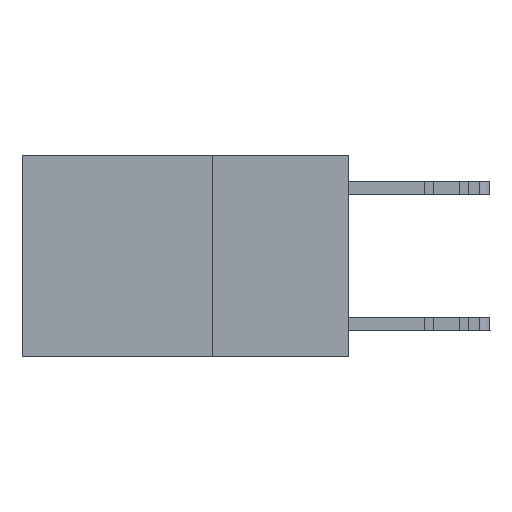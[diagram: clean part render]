
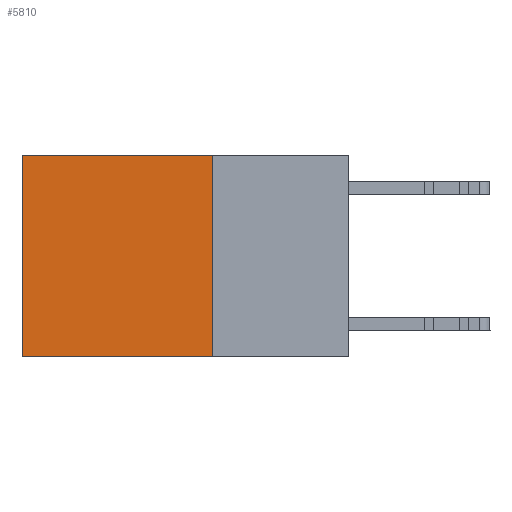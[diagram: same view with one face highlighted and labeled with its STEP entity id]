
A CAD part, left-side view. The second image highlights one B-rep face of the part: STEP entity #5810.
In plain terms, the highlighted planar face has unit normal (-1, 0, 0).
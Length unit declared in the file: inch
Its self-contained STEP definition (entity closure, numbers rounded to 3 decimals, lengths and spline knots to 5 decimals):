
#1325 = ORIENTED_EDGE ( 'NONE', *, *, #4437, .F. ) ;
#2714 = VERTEX_POINT ( 'NONE', #28033 ) ;
#4437 = EDGE_CURVE ( 'NONE', #5940, #8007, #23654, .T. ) ;
#5562 = CARTESIAN_POINT ( 'NONE',  ( 0.2625, 0.6, -0.37 ) ) ;
#5810 = ADVANCED_FACE ( 'NONE', ( #6890 ), #9930, .F. ) ;
#5861 = DIRECTION ( 'NONE',  ( 0., 0., -1. ) ) ;
#5940 = VERTEX_POINT ( 'NONE', #23942 ) ;
#6042 = DIRECTION ( 'NONE',  ( 1., 0., 0. ) ) ;
#6890 = FACE_OUTER_BOUND ( 'NONE', #17644, .T. ) ;
#8007 = VERTEX_POINT ( 'NONE', #5562 ) ;
#8303 = CARTESIAN_POINT ( 'NONE',  ( 0.2625, 0.25, 0. ) ) ;
#9930 = PLANE ( 'NONE',  #19287 ) ;
#10424 = LINE ( 'NONE', #21560, #10530 ) ;
#10530 = VECTOR ( 'NONE', #17144, 39.37008 ) ;
#12649 = EDGE_CURVE ( 'NONE', #2714, #5940, #20959, .T. ) ;
#12676 = VERTEX_POINT ( 'NONE', #23546 ) ;
#14909 = EDGE_CURVE ( 'NONE', #2714, #12676, #25557, .T. ) ;
#16536 = CARTESIAN_POINT ( 'NONE',  ( 0.2625, 0.25, -0.37 ) ) ;
#16691 = DIRECTION ( 'NONE',  ( 0., 1., 0. ) ) ;
#17123 = ORIENTED_EDGE ( 'NONE', *, *, #14909, .T. ) ;
#17144 = DIRECTION ( 'NONE',  ( 0., 0., -1. ) ) ;
#17644 = EDGE_LOOP ( 'NONE', ( #20929, #1325, #22571, #17123 ) ) ;
#18832 = DIRECTION ( 'NONE',  ( 0., 1., 0. ) ) ;
#18970 = CARTESIAN_POINT ( 'NONE',  ( 0.2625, 0.25, 0. ) ) ;
#19287 = AXIS2_PLACEMENT_3D ( 'NONE', #8303, #6042, #5861 ) ;
#20880 = VECTOR ( 'NONE', #24207, 39.37008 ) ;
#20929 = ORIENTED_EDGE ( 'NONE', *, *, #21820, .T. ) ;
#20959 = LINE ( 'NONE', #23978, #20880 ) ;
#21560 = CARTESIAN_POINT ( 'NONE',  ( 0.2625, 0.6, 0. ) ) ;
#21820 = EDGE_CURVE ( 'NONE', #12676, #8007, #10424, .T. ) ;
#22571 = ORIENTED_EDGE ( 'NONE', *, *, #12649, .F. ) ;
#23409 = VECTOR ( 'NONE', #16691, 39.37008 ) ;
#23534 = VECTOR ( 'NONE', #18832, 39.37008 ) ;
#23546 = CARTESIAN_POINT ( 'NONE',  ( 0.2625, 0.6, 0. ) ) ;
#23654 = LINE ( 'NONE', #16536, #23409 ) ;
#23942 = CARTESIAN_POINT ( 'NONE',  ( 0.2625, 0.25, -0.37 ) ) ;
#23978 = CARTESIAN_POINT ( 'NONE',  ( 0.2625, 0.25, 0. ) ) ;
#24207 = DIRECTION ( 'NONE',  ( 0., 0., -1. ) ) ;
#25557 = LINE ( 'NONE', #18970, #23534 ) ;
#28033 = CARTESIAN_POINT ( 'NONE',  ( 0.2625, 0.25, 0. ) ) ;
